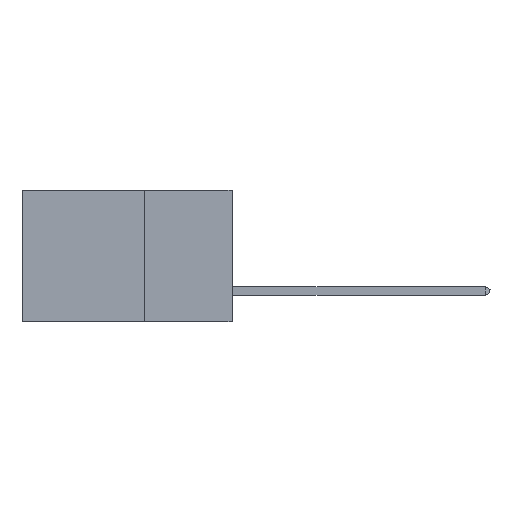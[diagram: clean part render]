
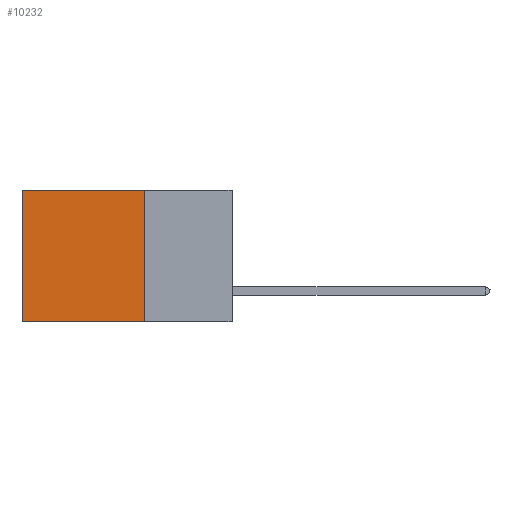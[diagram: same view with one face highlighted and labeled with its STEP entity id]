
A CAD part, left-side view. The second image highlights one B-rep face of the part: STEP entity #10232.
In plain terms, the highlighted planar face has unit normal (-1, 0, 0).
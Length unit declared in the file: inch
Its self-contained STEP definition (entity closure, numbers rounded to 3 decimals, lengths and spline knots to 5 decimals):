
#56 = DIRECTION ( 'NONE',  ( 0., 0., -1. ) ) ;
#707 = DIRECTION ( 'NONE',  ( 0., 1., 0. ) ) ;
#778 = LINE ( 'NONE', #7236, #9379 ) ;
#2206 = CARTESIAN_POINT ( 'NONE',  ( 0.2875, 0.25, -0.375 ) ) ;
#3089 = DIRECTION ( 'NONE',  ( 1., 0., 0. ) ) ;
#3179 = LINE ( 'NONE', #6505, #5668 ) ;
#4181 = PLANE ( 'NONE',  #7823 ) ;
#4416 = VERTEX_POINT ( 'NONE', #10165 ) ;
#4422 = CARTESIAN_POINT ( 'NONE',  ( 0.2875, 0.6, -0.375 ) ) ;
#4678 = VERTEX_POINT ( 'NONE', #14021 ) ;
#4789 = EDGE_LOOP ( 'NONE', ( #9689, #11859, #6262, #7265 ) ) ;
#5191 = VECTOR ( 'NONE', #9999, 39.37008 ) ;
#5635 = DIRECTION ( 'NONE',  ( 0., 1., 0. ) ) ;
#5668 = VECTOR ( 'NONE', #5635, 39.37008 ) ;
#6029 = EDGE_CURVE ( 'NONE', #4678, #7588, #10019, .T. ) ;
#6085 = VERTEX_POINT ( 'NONE', #6588 ) ;
#6262 = ORIENTED_EDGE ( 'NONE', *, *, #11628, .F. ) ;
#6464 = EDGE_CURVE ( 'NONE', #6085, #7588, #778, .T. ) ;
#6505 = CARTESIAN_POINT ( 'NONE',  ( 0.2875, 0.25, 0. ) ) ;
#6552 = EDGE_CURVE ( 'NONE', #4416, #4678, #3179, .T. ) ;
#6588 = CARTESIAN_POINT ( 'NONE',  ( 0.2875, 0.25, -0.375 ) ) ;
#6956 = CARTESIAN_POINT ( 'NONE',  ( 0.2875, 0.6, -0.375 ) ) ;
#7236 = CARTESIAN_POINT ( 'NONE',  ( 0.2875, 0.25, -0.375 ) ) ;
#7265 = ORIENTED_EDGE ( 'NONE', *, *, #6552, .T. ) ;
#7588 = VERTEX_POINT ( 'NONE', #6956 ) ;
#7823 = AXIS2_PLACEMENT_3D ( 'NONE', #11879, #3089, #8614 ) ;
#8614 = DIRECTION ( 'NONE',  ( 0., 0., -1. ) ) ;
#9052 = LINE ( 'NONE', #2206, #5191 ) ;
#9379 = VECTOR ( 'NONE', #707, 39.37008 ) ;
#9689 = ORIENTED_EDGE ( 'NONE', *, *, #6029, .T. ) ;
#9999 = DIRECTION ( 'NONE',  ( 0., 0., -1. ) ) ;
#10019 = LINE ( 'NONE', #4422, #13550 ) ;
#10165 = CARTESIAN_POINT ( 'NONE',  ( 0.2875, 0.25, 0. ) ) ;
#10232 = ADVANCED_FACE ( 'NONE', ( #10719 ), #4181, .F. ) ;
#10719 = FACE_OUTER_BOUND ( 'NONE', #4789, .T. ) ;
#11628 = EDGE_CURVE ( 'NONE', #4416, #6085, #9052, .T. ) ;
#11859 = ORIENTED_EDGE ( 'NONE', *, *, #6464, .F. ) ;
#11879 = CARTESIAN_POINT ( 'NONE',  ( 0.2875, 0.25, -0.375 ) ) ;
#13550 = VECTOR ( 'NONE', #56, 39.37008 ) ;
#14021 = CARTESIAN_POINT ( 'NONE',  ( 0.2875, 0.6, 0. ) ) ;
